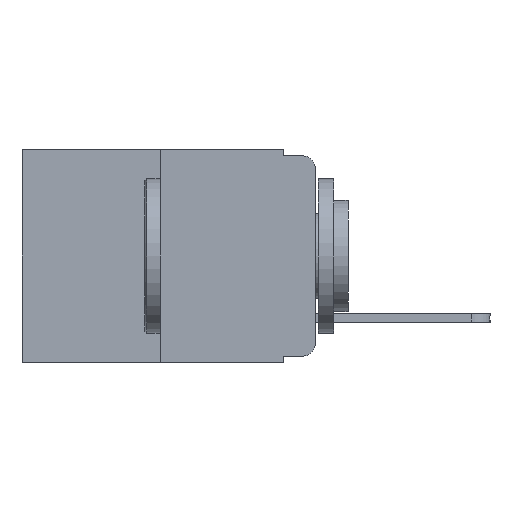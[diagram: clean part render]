
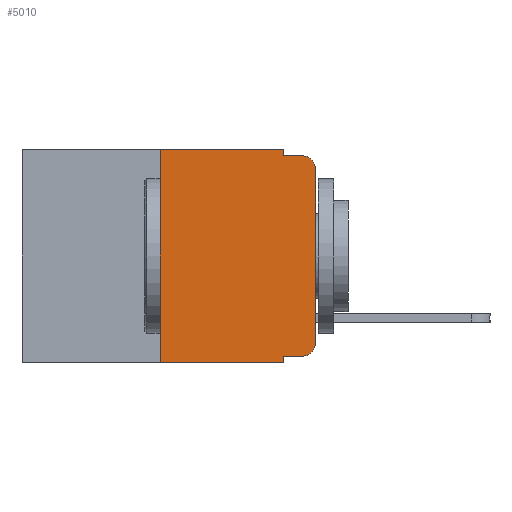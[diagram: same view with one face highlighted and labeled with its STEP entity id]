
A CAD part, left-side view. The second image highlights one B-rep face of the part: STEP entity #5010.
In plain terms, the highlighted planar face has unit normal (-1, 0, 0).
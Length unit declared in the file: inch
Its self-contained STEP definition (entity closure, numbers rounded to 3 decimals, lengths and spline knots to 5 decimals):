
#419 = LINE ( 'NONE', #17493, #3458 ) ;
#806 = CARTESIAN_POINT ( 'NONE',  ( 0., 0.473, -0.343 ) ) ;
#1061 = EDGE_CURVE ( 'NONE', #6570, #5754, #8854, .T. ) ;
#1461 = VERTEX_POINT ( 'NONE', #7425 ) ;
#1632 = VERTEX_POINT ( 'NONE', #14925 ) ;
#1937 = LINE ( 'NONE', #8443, #5582 ) ;
#2162 = EDGE_CURVE ( 'NONE', #5754, #1632, #1937, .T. ) ;
#2628 = VERTEX_POINT ( 'NONE', #16018 ) ;
#2743 = VECTOR ( 'NONE', #5110, 39.37008 ) ;
#2971 = VERTEX_POINT ( 'NONE', #3753 ) ;
#2997 = CARTESIAN_POINT ( 'NONE',  ( 0., 0.051, 0. ) ) ;
#3074 = DIRECTION ( 'NONE',  ( 0., 0., -1. ) ) ;
#3392 = DIRECTION ( 'NONE',  ( 0., 0., 1. ) ) ;
#3458 = VECTOR ( 'NONE', #9936, 39.37008 ) ;
#3475 = VECTOR ( 'NONE', #3074, 39.37008 ) ;
#3586 = EDGE_CURVE ( 'NONE', #16884, #4985, #12613, .T. ) ;
#3753 = CARTESIAN_POINT ( 'NONE',  ( 0., 0.051, -0.01 ) ) ;
#3951 = LINE ( 'NONE', #2997, #3475 ) ;
#4036 = ORIENTED_EDGE ( 'NONE', *, *, #3586, .T. ) ;
#4667 = VECTOR ( 'NONE', #3392, 39.37008 ) ;
#4985 = VERTEX_POINT ( 'NONE', #6665 ) ;
#5010 = ADVANCED_FACE ( 'NONE', ( #14698 ), #14820, .F. ) ;
#5110 = DIRECTION ( 'NONE',  ( 0., -1., 0. ) ) ;
#5181 = CARTESIAN_POINT ( 'NONE',  ( 0., 0., -0.03 ) ) ;
#5552 = EDGE_CURVE ( 'NONE', #6570, #8220, #8695, .T. ) ;
#5582 = VECTOR ( 'NONE', #8623, 39.37008 ) ;
#5754 = VERTEX_POINT ( 'NONE', #9402 ) ;
#5907 = DIRECTION ( 'NONE',  ( 0., 0., -1. ) ) ;
#5914 = EDGE_CURVE ( 'NONE', #8719, #2628, #6434, .T. ) ;
#6168 = CARTESIAN_POINT ( 'NONE',  ( 0., 0.25, -0.343 ) ) ;
#6260 = CARTESIAN_POINT ( 'NONE',  ( 0., 0.02, -0.03 ) ) ;
#6268 = ORIENTED_EDGE ( 'NONE', *, *, #11911, .T. ) ;
#6434 = CIRCLE ( 'NONE', #14762, 0.02 ) ;
#6455 = CARTESIAN_POINT ( 'NONE',  ( 0., 0.473, 0. ) ) ;
#6570 = VERTEX_POINT ( 'NONE', #6168 ) ;
#6665 = CARTESIAN_POINT ( 'NONE',  ( 0., 0., -0.313 ) ) ;
#7191 = CARTESIAN_POINT ( 'NONE',  ( 0., 0.02, -0.333 ) ) ;
#7425 = CARTESIAN_POINT ( 'NONE',  ( 0., 0.051, -0.333 ) ) ;
#7681 = ORIENTED_EDGE ( 'NONE', *, *, #10881, .F. ) ;
#7868 = DIRECTION ( 'NONE',  ( 0., 0., -1. ) ) ;
#7994 = DIRECTION ( 'NONE',  ( 0., -1., 0. ) ) ;
#8220 = VERTEX_POINT ( 'NONE', #9094 ) ;
#8311 = AXIS2_PLACEMENT_3D ( 'NONE', #14671, #16546, #16528 ) ;
#8443 = CARTESIAN_POINT ( 'NONE',  ( 0., 0.473, 0. ) ) ;
#8623 = DIRECTION ( 'NONE',  ( 0., -1., 0. ) ) ;
#8695 = LINE ( 'NONE', #806, #16333 ) ;
#8704 = ORIENTED_EDGE ( 'NONE', *, *, #2162, .F. ) ;
#8719 = VERTEX_POINT ( 'NONE', #5181 ) ;
#8854 = LINE ( 'NONE', #15167, #4667 ) ;
#8996 = ORIENTED_EDGE ( 'NONE', *, *, #1061, .F. ) ;
#9094 = CARTESIAN_POINT ( 'NONE',  ( 0., 0.051, -0.343 ) ) ;
#9124 = ORIENTED_EDGE ( 'NONE', *, *, #5552, .T. ) ;
#9402 = CARTESIAN_POINT ( 'NONE',  ( 0., 0.25, 0. ) ) ;
#9631 = ORIENTED_EDGE ( 'NONE', *, *, #15354, .F. ) ;
#9936 = DIRECTION ( 'NONE',  ( 0., 0., 1. ) ) ;
#10881 = EDGE_CURVE ( 'NONE', #1632, #2971, #3951, .T. ) ;
#11129 = ORIENTED_EDGE ( 'NONE', *, *, #11274, .F. ) ;
#11213 = EDGE_LOOP ( 'NONE', ( #6268, #16969, #11129, #7681, #8704, #8996, #9124, #9631, #18485, #4036 ) ) ;
#11274 = EDGE_CURVE ( 'NONE', #2971, #2628, #12203, .T. ) ;
#11820 = CARTESIAN_POINT ( 'NONE',  ( 0., 0.051, -0.01 ) ) ;
#11911 = EDGE_CURVE ( 'NONE', #4985, #8719, #419, .T. ) ;
#11982 = VECTOR ( 'NONE', #5907, 39.37008 ) ;
#12203 = LINE ( 'NONE', #11820, #19751 ) ;
#12613 = CIRCLE ( 'NONE', #8311, 0.02 ) ;
#12851 = CARTESIAN_POINT ( 'NONE',  ( 0., 0.051, -0.333 ) ) ;
#13252 = DIRECTION ( 'NONE',  ( 0., 0., -1. ) ) ;
#13355 = DIRECTION ( 'NONE',  ( 0., -1., 0. ) ) ;
#13652 = CARTESIAN_POINT ( 'NONE',  ( 0., 0.051, 0. ) ) ;
#14671 = CARTESIAN_POINT ( 'NONE',  ( 0., 0.02, -0.313 ) ) ;
#14698 = FACE_OUTER_BOUND ( 'NONE', #11213, .T. ) ;
#14756 = DIRECTION ( 'NONE',  ( 1., 0., 0. ) ) ;
#14762 = AXIS2_PLACEMENT_3D ( 'NONE', #6260, #17030, #7868 ) ;
#14820 = PLANE ( 'NONE',  #15904 ) ;
#14925 = CARTESIAN_POINT ( 'NONE',  ( 0., 0.051, 0. ) ) ;
#14974 = EDGE_CURVE ( 'NONE', #1461, #16884, #19093, .T. ) ;
#15167 = CARTESIAN_POINT ( 'NONE',  ( 0., 0.25, 0. ) ) ;
#15354 = EDGE_CURVE ( 'NONE', #1461, #8220, #20006, .T. ) ;
#15904 = AXIS2_PLACEMENT_3D ( 'NONE', #6455, #14756, #13252 ) ;
#16018 = CARTESIAN_POINT ( 'NONE',  ( 0., 0.02, -0.01 ) ) ;
#16333 = VECTOR ( 'NONE', #7994, 39.37008 ) ;
#16528 = DIRECTION ( 'NONE',  ( 0., 0., -1. ) ) ;
#16546 = DIRECTION ( 'NONE',  ( -1., 0., 0. ) ) ;
#16884 = VERTEX_POINT ( 'NONE', #7191 ) ;
#16969 = ORIENTED_EDGE ( 'NONE', *, *, #5914, .T. ) ;
#17030 = DIRECTION ( 'NONE',  ( -1., 0., 0. ) ) ;
#17493 = CARTESIAN_POINT ( 'NONE',  ( 0., 0., 0. ) ) ;
#18485 = ORIENTED_EDGE ( 'NONE', *, *, #14974, .T. ) ;
#19093 = LINE ( 'NONE', #12851, #2743 ) ;
#19751 = VECTOR ( 'NONE', #13355, 39.37008 ) ;
#20006 = LINE ( 'NONE', #13652, #11982 ) ;
